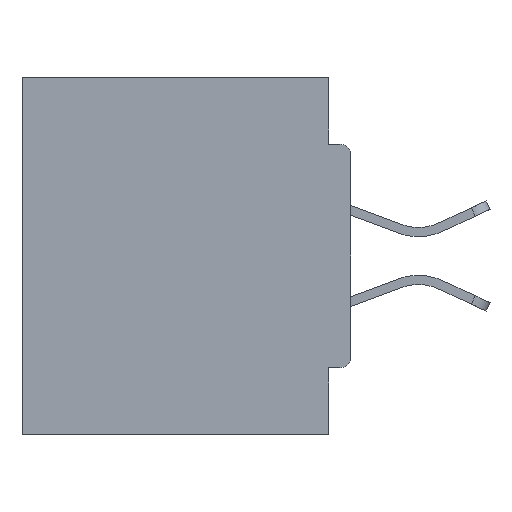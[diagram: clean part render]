
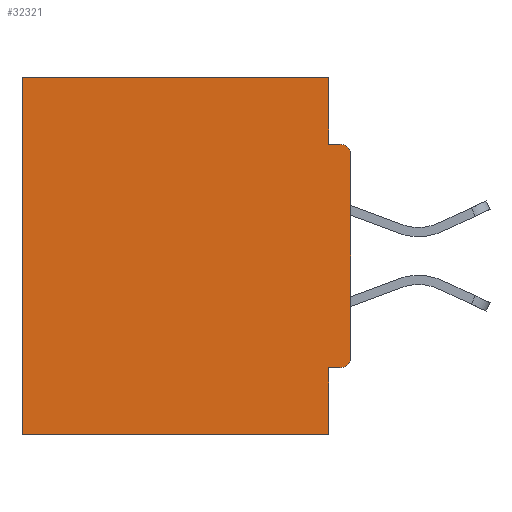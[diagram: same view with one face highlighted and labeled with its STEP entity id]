
A CAD part, left-side view. The second image highlights one B-rep face of the part: STEP entity #32321.
In plain terms, the highlighted planar face has unit normal (-1, 0, 0).
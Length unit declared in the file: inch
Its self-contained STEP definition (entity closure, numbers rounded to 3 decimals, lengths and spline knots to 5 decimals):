
#599 = CARTESIAN_POINT ( 'NONE',  ( 0.298, 0., -0.4065 ) ) ;
#624 = CARTESIAN_POINT ( 'NONE',  ( 0.298, 0.015, -0.3915 ) ) ;
#1044 = DIRECTION ( 'NONE',  ( 1., 0., 0. ) ) ;
#1421 = CARTESIAN_POINT ( 'NONE',  ( 0.298, 0., -0.5 ) ) ;
#1953 = LINE ( 'NONE', #6168, #34337 ) ;
#2466 = AXIS2_PLACEMENT_3D ( 'NONE', #22187, #1044, #3512 ) ;
#2553 = DIRECTION ( 'NONE',  ( 0., 0., -1. ) ) ;
#3040 = AXIS2_PLACEMENT_3D ( 'NONE', #21593, #26714, #16199 ) ;
#3287 = ORIENTED_EDGE ( 'NONE', *, *, #33508, .F. ) ;
#3380 = VECTOR ( 'NONE', #32798, 39.37008 ) ;
#3512 = DIRECTION ( 'NONE',  ( 0., 0., -1. ) ) ;
#3781 = CARTESIAN_POINT ( 'NONE',  ( 0.298, 0.031, -0.5 ) ) ;
#4130 = CARTESIAN_POINT ( 'NONE',  ( 0.298, 0.46, 0. ) ) ;
#4134 = DIRECTION ( 'NONE',  ( 0., 1., 0. ) ) ;
#4508 = EDGE_CURVE ( 'NONE', #24175, #23217, #34450, .T. ) ;
#5412 = VERTEX_POINT ( 'NONE', #4130 ) ;
#5726 = CARTESIAN_POINT ( 'NONE',  ( 0.298, 0.031, -0.0935 ) ) ;
#6168 = CARTESIAN_POINT ( 'NONE',  ( 0.298, 0.46, 0. ) ) ;
#6417 = LINE ( 'NONE', #1421, #21944 ) ;
#7356 = ORIENTED_EDGE ( 'NONE', *, *, #4508, .F. ) ;
#7805 = VECTOR ( 'NONE', #20217, 39.37008 ) ;
#7927 = CARTESIAN_POINT ( 'NONE',  ( 0.298, 0., -0.1085 ) ) ;
#8017 = EDGE_CURVE ( 'NONE', #5412, #22107, #1953, .T. ) ;
#8654 = CARTESIAN_POINT ( 'NONE',  ( 0.298, 0., 0. ) ) ;
#8685 = PLANE ( 'NONE',  #2466 ) ;
#9413 = VERTEX_POINT ( 'NONE', #14261 ) ;
#10295 = CARTESIAN_POINT ( 'NONE',  ( 0.298, 0.031, -0.4065 ) ) ;
#10512 = LINE ( 'NONE', #599, #3380 ) ;
#11215 = ORIENTED_EDGE ( 'NONE', *, *, #26581, .F. ) ;
#11689 = ORIENTED_EDGE ( 'NONE', *, *, #11997, .T. ) ;
#11997 = EDGE_CURVE ( 'NONE', #29093, #5412, #15623, .T. ) ;
#12088 = ORIENTED_EDGE ( 'NONE', *, *, #8017, .T. ) ;
#12467 = VERTEX_POINT ( 'NONE', #17122 ) ;
#12544 = ORIENTED_EDGE ( 'NONE', *, *, #27831, .T. ) ;
#13478 = CARTESIAN_POINT ( 'NONE',  ( 0.298, 0.031, -0.5 ) ) ;
#14035 = DIRECTION ( 'NONE',  ( 0., 0., -1. ) ) ;
#14261 = CARTESIAN_POINT ( 'NONE',  ( 0.298, 0.015, -0.0935 ) ) ;
#14332 = ORIENTED_EDGE ( 'NONE', *, *, #24541, .F. ) ;
#15623 = LINE ( 'NONE', #15965, #21507 ) ;
#15965 = CARTESIAN_POINT ( 'NONE',  ( 0.298, 0., 0. ) ) ;
#16199 = DIRECTION ( 'NONE',  ( 0., 0., -1. ) ) ;
#16552 = DIRECTION ( 'NONE',  ( 0., 0., -1. ) ) ;
#16867 = DIRECTION ( 'NONE',  ( -1., 0., 0. ) ) ;
#17122 = CARTESIAN_POINT ( 'NONE',  ( 0.298, 0.015, -0.4065 ) ) ;
#17245 = VECTOR ( 'NONE', #16552, 39.37008 ) ;
#18396 = CARTESIAN_POINT ( 'NONE',  ( 0.298, 0.031, -0.5 ) ) ;
#18644 = CIRCLE ( 'NONE', #24244, 0.015 ) ;
#18673 = DIRECTION ( 'NONE',  ( 0., 1., 0. ) ) ;
#19550 = EDGE_CURVE ( 'NONE', #28630, #22107, #6417, .T. ) ;
#20177 = DIRECTION ( 'NONE',  ( 0., -1., 0. ) ) ;
#20217 = DIRECTION ( 'NONE',  ( 0., 0., -1. ) ) ;
#20622 = CARTESIAN_POINT ( 'NONE',  ( 0.298, 0., -0.0935 ) ) ;
#21164 = EDGE_LOOP ( 'NONE', ( #12544, #14332, #22713, #11689, #12088, #27457, #3287, #11215, #34652, #7356 ) ) ;
#21507 = VECTOR ( 'NONE', #18673, 39.37008 ) ;
#21593 = CARTESIAN_POINT ( 'NONE',  ( 0.298, 0.015, -0.1085 ) ) ;
#21662 = VERTEX_POINT ( 'NONE', #10295 ) ;
#21664 = CARTESIAN_POINT ( 'NONE',  ( 0.298, 0., -0.3915 ) ) ;
#21944 = VECTOR ( 'NONE', #4134, 39.37008 ) ;
#22107 = VERTEX_POINT ( 'NONE', #31054 ) ;
#22187 = CARTESIAN_POINT ( 'NONE',  ( 0.298, 0., 0. ) ) ;
#22713 = ORIENTED_EDGE ( 'NONE', *, *, #30640, .F. ) ;
#23217 = VERTEX_POINT ( 'NONE', #21664 ) ;
#24006 = LINE ( 'NONE', #13478, #29439 ) ;
#24175 = VERTEX_POINT ( 'NONE', #7927 ) ;
#24244 = AXIS2_PLACEMENT_3D ( 'NONE', #624, #16867, #14035 ) ;
#24541 = EDGE_CURVE ( 'NONE', #32829, #9413, #34575, .T. ) ;
#26272 = LINE ( 'NONE', #3781, #7805 ) ;
#26581 = EDGE_CURVE ( 'NONE', #12467, #21662, #10512, .T. ) ;
#26714 = DIRECTION ( 'NONE',  ( -1., 0., 0. ) ) ;
#27421 = VECTOR ( 'NONE', #20177, 39.37008 ) ;
#27457 = ORIENTED_EDGE ( 'NONE', *, *, #19550, .F. ) ;
#27648 = DIRECTION ( 'NONE',  ( 0., 0., -1. ) ) ;
#27831 = EDGE_CURVE ( 'NONE', #24175, #9413, #34378, .T. ) ;
#28630 = VERTEX_POINT ( 'NONE', #18396 ) ;
#29093 = VERTEX_POINT ( 'NONE', #31703 ) ;
#29439 = VECTOR ( 'NONE', #2553, 39.37008 ) ;
#30012 = EDGE_CURVE ( 'NONE', #12467, #23217, #18644, .T. ) ;
#30640 = EDGE_CURVE ( 'NONE', #29093, #32829, #24006, .T. ) ;
#31054 = CARTESIAN_POINT ( 'NONE',  ( 0.298, 0.46, -0.5 ) ) ;
#31703 = CARTESIAN_POINT ( 'NONE',  ( 0.298, 0.031, 0. ) ) ;
#32321 = ADVANCED_FACE ( 'NONE', ( #34403 ), #8685, .F. ) ;
#32798 = DIRECTION ( 'NONE',  ( 0., 1., 0. ) ) ;
#32829 = VERTEX_POINT ( 'NONE', #5726 ) ;
#33508 = EDGE_CURVE ( 'NONE', #21662, #28630, #26272, .T. ) ;
#34337 = VECTOR ( 'NONE', #27648, 39.37008 ) ;
#34378 = CIRCLE ( 'NONE', #3040, 0.015 ) ;
#34403 = FACE_OUTER_BOUND ( 'NONE', #21164, .T. ) ;
#34450 = LINE ( 'NONE', #8654, #17245 ) ;
#34575 = LINE ( 'NONE', #20622, #27421 ) ;
#34652 = ORIENTED_EDGE ( 'NONE', *, *, #30012, .T. ) ;
